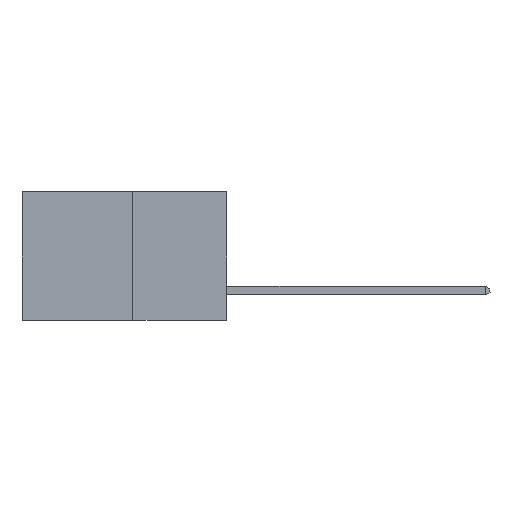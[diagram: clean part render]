
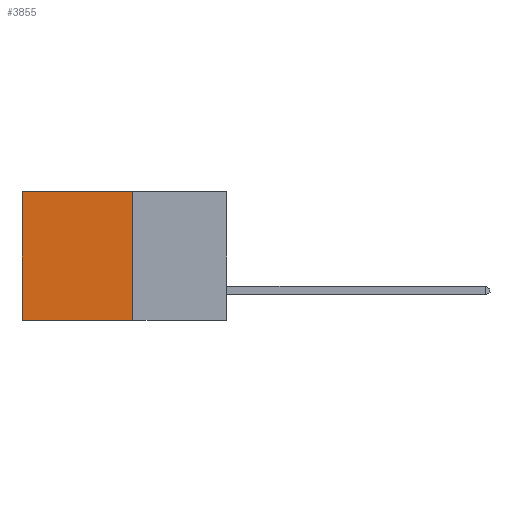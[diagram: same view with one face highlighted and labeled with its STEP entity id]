
A CAD part, left-side view. The second image highlights one B-rep face of the part: STEP entity #3855.
In plain terms, the highlighted planar face has unit normal (-1, 0, 0).
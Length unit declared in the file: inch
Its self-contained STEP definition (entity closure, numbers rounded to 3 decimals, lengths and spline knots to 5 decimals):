
#518 = ORIENTED_EDGE ( 'NONE', *, *, #1264, .T. ) ;
#618 = ORIENTED_EDGE ( 'NONE', *, *, #11020, .F. ) ;
#793 = ORIENTED_EDGE ( 'NONE', *, *, #7200, .F. ) ;
#795 = DIRECTION ( 'NONE',  ( 0., 1., 0. ) ) ;
#813 = ORIENTED_EDGE ( 'NONE', *, *, #3632, .T. ) ;
#1264 = EDGE_CURVE ( 'NONE', #8258, #2319, #5658, .T. ) ;
#1334 = LINE ( 'NONE', #2726, #10809 ) ;
#2319 = VERTEX_POINT ( 'NONE', #7354 ) ;
#2726 = CARTESIAN_POINT ( 'NONE',  ( 0.277, 0.27, 0. ) ) ;
#3632 = EDGE_CURVE ( 'NONE', #11761, #8258, #1334, .T. ) ;
#3701 = CARTESIAN_POINT ( 'NONE',  ( 0.277, 0.27, -0.37 ) ) ;
#3855 = ADVANCED_FACE ( 'NONE', ( #6209 ), #6245, .F. ) ;
#4039 = CARTESIAN_POINT ( 'NONE',  ( 0.277, 0.59, -0.37 ) ) ;
#4381 = AXIS2_PLACEMENT_3D ( 'NONE', #5623, #6194, #5296 ) ;
#4887 = LINE ( 'NONE', #11587, #9294 ) ;
#5296 = DIRECTION ( 'NONE',  ( 0., 0., -1. ) ) ;
#5404 = CARTESIAN_POINT ( 'NONE',  ( 0.277, 0.27, 0. ) ) ;
#5623 = CARTESIAN_POINT ( 'NONE',  ( 0.277, 0.27, -0.37 ) ) ;
#5658 = LINE ( 'NONE', #4039, #9950 ) ;
#6015 = CARTESIAN_POINT ( 'NONE',  ( 0.277, 0.27, -0.37 ) ) ;
#6194 = DIRECTION ( 'NONE',  ( 1., 0., 0. ) ) ;
#6209 = FACE_OUTER_BOUND ( 'NONE', #7471, .T. ) ;
#6245 = PLANE ( 'NONE',  #4381 ) ;
#6763 = VECTOR ( 'NONE', #795, 39.37008 ) ;
#7020 = LINE ( 'NONE', #3701, #6763 ) ;
#7200 = EDGE_CURVE ( 'NONE', #11761, #9583, #4887, .T. ) ;
#7354 = CARTESIAN_POINT ( 'NONE',  ( 0.277, 0.59, -0.37 ) ) ;
#7471 = EDGE_LOOP ( 'NONE', ( #518, #618, #793, #813 ) ) ;
#8258 = VERTEX_POINT ( 'NONE', #10805 ) ;
#9294 = VECTOR ( 'NONE', #11208, 39.37008 ) ;
#9583 = VERTEX_POINT ( 'NONE', #6015 ) ;
#9950 = VECTOR ( 'NONE', #10395, 39.37008 ) ;
#10395 = DIRECTION ( 'NONE',  ( 0., 0., -1. ) ) ;
#10805 = CARTESIAN_POINT ( 'NONE',  ( 0.277, 0.59, 0. ) ) ;
#10809 = VECTOR ( 'NONE', #11511, 39.37008 ) ;
#11020 = EDGE_CURVE ( 'NONE', #9583, #2319, #7020, .T. ) ;
#11208 = DIRECTION ( 'NONE',  ( 0., 0., -1. ) ) ;
#11511 = DIRECTION ( 'NONE',  ( 0., 1., 0. ) ) ;
#11587 = CARTESIAN_POINT ( 'NONE',  ( 0.277, 0.27, -0.37 ) ) ;
#11761 = VERTEX_POINT ( 'NONE', #5404 ) ;
